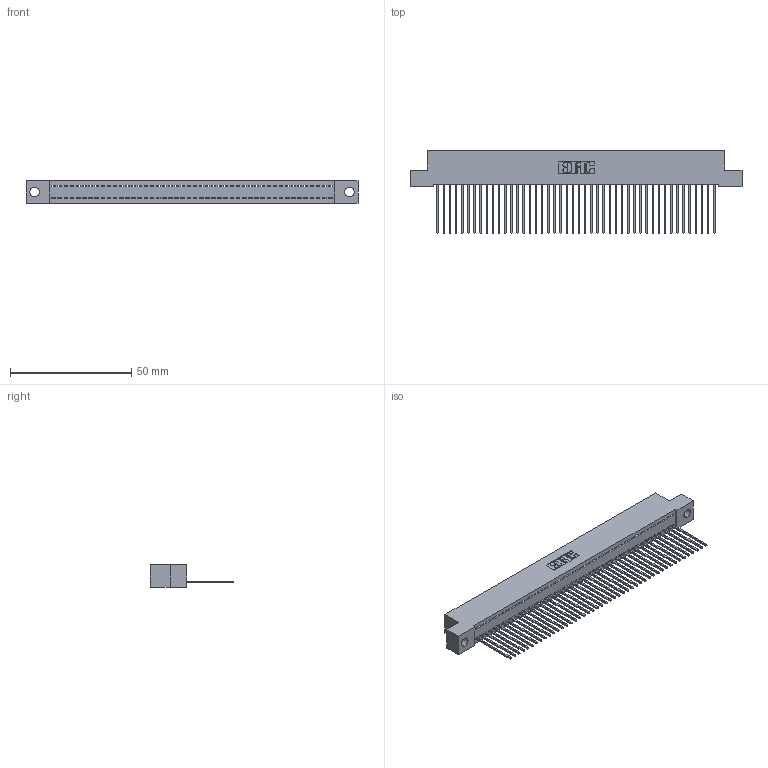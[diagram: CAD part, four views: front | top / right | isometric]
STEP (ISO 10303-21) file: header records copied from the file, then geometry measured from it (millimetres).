
FILE_DESCRIPTION (( 'STEP AP203' ), '1' );
FILE_NAME ('392-046-541-104.STEP', '2018-08-16T16:54:04', ( '' ), ( '' ), 'SwSTEP 2.0', 'SolidWorks 2016', '' );
FILE_SCHEMA (( 'CONFIG_CONTROL_DESIGN' ));
Length unit declared in the file: inch
Products named in the file (3): 342 Part_.156 TH; 345-292-001_345-293-141; 392-046-541-104
Assembly tree (47 placements, depth 2):
  392-046-541-104
    342 Part_.156 TH
    345-292-001_345-293-141  x46
Bounding box: 137.16 x 34.3 x 9.4 mm (x, y, z)
Volume: 12105.7 mm3; surface area: 18533.3 mm2
Topology: 47 solids, 47 shells, 2778 faces, 8395 edges, 5534 vertices
Faces by surface type: plane 1998, cylinder 780
Entity records: 27493 total; most frequent: CARTESIAN_POINT 4748, ORIENTED_EDGE 4730, DIRECTION 3997, EDGE_CURVE 2365, VECTOR 2237, LINE 2237, VERTEX_POINT 1574, AXIS2_PLACEMENT_3D 880
